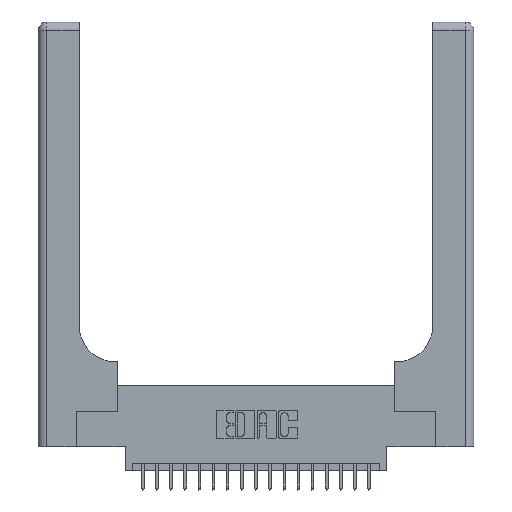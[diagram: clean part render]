
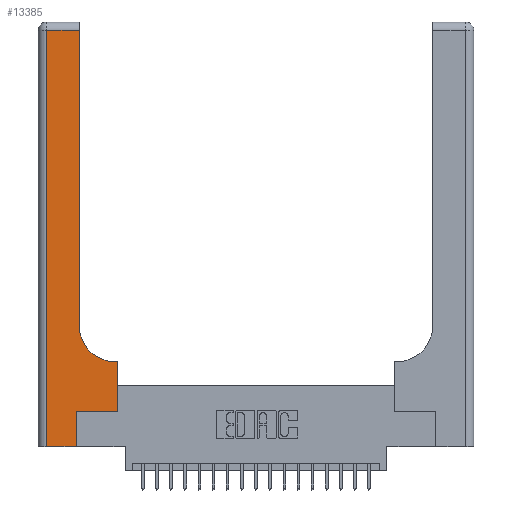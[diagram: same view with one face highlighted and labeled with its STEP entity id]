
A CAD part, top view. The second image highlights one B-rep face of the part: STEP entity #13385.
In plain terms, the highlighted planar face has unit normal (0, 0, 1).
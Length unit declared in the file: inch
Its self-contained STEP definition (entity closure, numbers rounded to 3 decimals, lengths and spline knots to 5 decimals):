
#221 = ORIENTED_EDGE ( 'NONE', *, *, #12865, .T. ) ;
#487 = VECTOR ( 'NONE', #12266, 39.37008 ) ;
#580 = VECTOR ( 'NONE', #916, 39.37008 ) ;
#916 = DIRECTION ( 'NONE',  ( -1., 0., 0. ) ) ;
#1025 = DIRECTION ( 'NONE',  ( -1., 0., 0. ) ) ;
#1036 = EDGE_LOOP ( 'NONE', ( #8035, #4315, #3704, #9746, #11403, #12290, #221, #9781, #21205 ) ) ;
#1178 = CARTESIAN_POINT ( 'NONE',  ( 0.5415, 0.85, 0.37 ) ) ;
#1473 = CARTESIAN_POINT ( 'NONE',  ( 0.5585, 0.6, 0.37 ) ) ;
#1574 = EDGE_CURVE ( 'NONE', #12773, #6876, #17489, .T. ) ;
#1803 = CARTESIAN_POINT ( 'NONE',  ( 0., 2.94, 0.37 ) ) ;
#2474 = LINE ( 'NONE', #12655, #580 ) ;
#3350 = DIRECTION ( 'NONE',  ( 1., 0., 0. ) ) ;
#3704 = ORIENTED_EDGE ( 'NONE', *, *, #4006, .T. ) ;
#3779 = CARTESIAN_POINT ( 'NONE',  ( 0.5585, 0.25, 0.37 ) ) ;
#3876 = CARTESIAN_POINT ( 'NONE',  ( 0.06, 0., 0.37 ) ) ;
#3977 = EDGE_CURVE ( 'NONE', #11319, #4254, #6774, .T. ) ;
#4006 = EDGE_CURVE ( 'NONE', #15480, #4893, #15114, .T. ) ;
#4254 = VERTEX_POINT ( 'NONE', #16209 ) ;
#4315 = ORIENTED_EDGE ( 'NONE', *, *, #18703, .T. ) ;
#4893 = VERTEX_POINT ( 'NONE', #3876 ) ;
#5056 = LINE ( 'NONE', #3779, #17757 ) ;
#5321 = AXIS2_PLACEMENT_3D ( 'NONE', #1178, #8049, #19901 ) ;
#5624 = CARTESIAN_POINT ( 'NONE',  ( 0.2915, 2.94, 0.37 ) ) ;
#5755 = DIRECTION ( 'NONE',  ( -1., 0., 0. ) ) ;
#5930 = DIRECTION ( 'NONE',  ( 0., 1., 0. ) ) ;
#6412 = VECTOR ( 'NONE', #14883, 39.37008 ) ;
#6455 = VECTOR ( 'NONE', #13354, 39.37008 ) ;
#6694 = CARTESIAN_POINT ( 'NONE',  ( 0.06, 3., 0.37 ) ) ;
#6774 = CIRCLE ( 'NONE', #5321, 0.25 ) ;
#6876 = VERTEX_POINT ( 'NONE', #21151 ) ;
#8035 = ORIENTED_EDGE ( 'NONE', *, *, #19330, .T. ) ;
#8049 = DIRECTION ( 'NONE',  ( 0., 0., -1. ) ) ;
#9714 = VECTOR ( 'NONE', #20502, 39.37008 ) ;
#9746 = ORIENTED_EDGE ( 'NONE', *, *, #10050, .T. ) ;
#9781 = ORIENTED_EDGE ( 'NONE', *, *, #13337, .T. ) ;
#10050 = EDGE_CURVE ( 'NONE', #4893, #16941, #18803, .T. ) ;
#10090 = CARTESIAN_POINT ( 'NONE',  ( 0.269, 0., 0.37 ) ) ;
#10447 = CARTESIAN_POINT ( 'NONE',  ( 0.269, 0.25, 0.37 ) ) ;
#10563 = CARTESIAN_POINT ( 'NONE',  ( 0.269, 0., 0.37 ) ) ;
#11319 = VERTEX_POINT ( 'NONE', #17722 ) ;
#11357 = VERTEX_POINT ( 'NONE', #5624 ) ;
#11403 = ORIENTED_EDGE ( 'NONE', *, *, #19187, .T. ) ;
#11449 = LINE ( 'NONE', #13240, #6455 ) ;
#12165 = VERTEX_POINT ( 'NONE', #1473 ) ;
#12266 = DIRECTION ( 'NONE',  ( 1., 0., 0. ) ) ;
#12290 = ORIENTED_EDGE ( 'NONE', *, *, #1574, .T. ) ;
#12542 = VECTOR ( 'NONE', #3350, 39.37008 ) ;
#12655 = CARTESIAN_POINT ( 'NONE',  ( 0.2915, 0.6, 0.37 ) ) ;
#12773 = VERTEX_POINT ( 'NONE', #10447 ) ;
#12865 = EDGE_CURVE ( 'NONE', #6876, #12165, #5056, .T. ) ;
#13240 = CARTESIAN_POINT ( 'NONE',  ( 0.2915, 3., 0.37 ) ) ;
#13337 = EDGE_CURVE ( 'NONE', #12165, #11319, #2474, .T. ) ;
#13354 = DIRECTION ( 'NONE',  ( 0., 1., 0. ) ) ;
#13385 = ADVANCED_FACE ( 'NONE', ( #14504 ), #14617, .F. ) ;
#14504 = FACE_OUTER_BOUND ( 'NONE', #1036, .T. ) ;
#14617 = PLANE ( 'NONE',  #17083 ) ;
#14883 = DIRECTION ( 'NONE',  ( 0., -1., 0. ) ) ;
#15114 = LINE ( 'NONE', #6694, #6412 ) ;
#15474 = CARTESIAN_POINT ( 'NONE',  ( 0., 0., 0.37 ) ) ;
#15480 = VERTEX_POINT ( 'NONE', #18789 ) ;
#15722 = LINE ( 'NONE', #1803, #19664 ) ;
#15927 = LINE ( 'NONE', #10563, #9714 ) ;
#16209 = CARTESIAN_POINT ( 'NONE',  ( 0.2915, 0.85, 0.37 ) ) ;
#16413 = DIRECTION ( 'NONE',  ( 0., 0., -1. ) ) ;
#16941 = VERTEX_POINT ( 'NONE', #10090 ) ;
#17083 = AXIS2_PLACEMENT_3D ( 'NONE', #18072, #16413, #1025 ) ;
#17489 = LINE ( 'NONE', #18813, #12542 ) ;
#17722 = CARTESIAN_POINT ( 'NONE',  ( 0.5415, 0.6, 0.37 ) ) ;
#17757 = VECTOR ( 'NONE', #5930, 39.37008 ) ;
#18072 = CARTESIAN_POINT ( 'NONE',  ( 0., 3., 0.37 ) ) ;
#18703 = EDGE_CURVE ( 'NONE', #11357, #15480, #15722, .T. ) ;
#18789 = CARTESIAN_POINT ( 'NONE',  ( 0.06, 2.94, 0.37 ) ) ;
#18803 = LINE ( 'NONE', #15474, #487 ) ;
#18813 = CARTESIAN_POINT ( 'NONE',  ( 0.269, 0.25, 0.37 ) ) ;
#19187 = EDGE_CURVE ( 'NONE', #16941, #12773, #15927, .T. ) ;
#19330 = EDGE_CURVE ( 'NONE', #4254, #11357, #11449, .T. ) ;
#19664 = VECTOR ( 'NONE', #5755, 39.37008 ) ;
#19901 = DIRECTION ( 'NONE',  ( 1., 0., 0. ) ) ;
#20502 = DIRECTION ( 'NONE',  ( 0., 1., 0. ) ) ;
#21151 = CARTESIAN_POINT ( 'NONE',  ( 0.5585, 0.25, 0.37 ) ) ;
#21205 = ORIENTED_EDGE ( 'NONE', *, *, #3977, .T. ) ;
